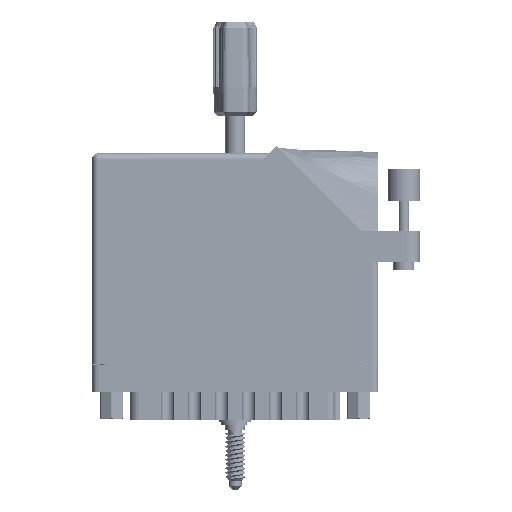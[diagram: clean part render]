
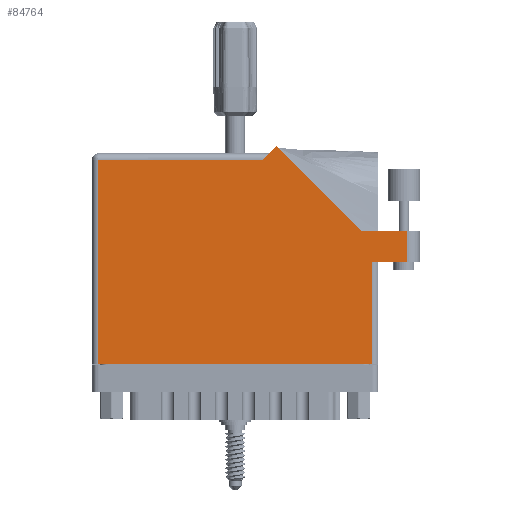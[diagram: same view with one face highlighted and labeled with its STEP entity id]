
A CAD part, front view. The second image highlights one B-rep face of the part: STEP entity #84764.
In plain terms, the highlighted face is planar.
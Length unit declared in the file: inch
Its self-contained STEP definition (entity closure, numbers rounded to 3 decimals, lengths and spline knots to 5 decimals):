
#1753 = CARTESIAN_POINT ( 'NONE',  ( 2.58942, 1.287, 0. ) ) ;
#4302 = EDGE_CURVE ( 'NONE', #12360, #84001, #58504, .T. ) ;
#6374 = LINE ( 'NONE', #61199, #70724 ) ;
#8116 = VERTEX_POINT ( 'NONE', #1753 ) ;
#9251 = VECTOR ( 'NONE', #90883, 39.37008 ) ;
#9544 = EDGE_CURVE ( 'NONE', #60245, #32958, #101732, .T. ) ;
#10695 = LINE ( 'NONE', #95578, #43067 ) ;
#12360 = VERTEX_POINT ( 'NONE', #118815 ) ;
#12663 = LINE ( 'NONE', #50572, #86017 ) ;
#13843 = CARTESIAN_POINT ( 'NONE',  ( 3.03, 0.98, 0. ) ) ;
#19299 = PLANE ( 'NONE',  #104740 ) ;
#20911 = CARTESIAN_POINT ( 'NONE',  ( 3.03, 1.287, 0. ) ) ;
#21012 = ORIENTED_EDGE ( 'NONE', *, *, #90095, .T. ) ;
#22523 = ORIENTED_EDGE ( 'NONE', *, *, #74579, .T. ) ;
#22728 = DIRECTION ( 'NONE',  ( 0., -1., 0. ) ) ;
#24081 = DIRECTION ( 'NONE',  ( 1., 0., 0. ) ) ;
#24288 = VECTOR ( 'NONE', #39299, 39.37008 ) ;
#24999 = VECTOR ( 'NONE', #111271, 39.37008 ) ;
#27294 = ORIENTED_EDGE ( 'NONE', *, *, #9544, .T. ) ;
#27380 = ORIENTED_EDGE ( 'NONE', *, *, #41243, .T. ) ;
#28600 = ORIENTED_EDGE ( 'NONE', *, *, #4302, .T. ) ;
#28712 = ORIENTED_EDGE ( 'NONE', *, *, #85772, .T. ) ;
#30125 = EDGE_CURVE ( 'NONE', #8116, #107748, #12663, .T. ) ;
#32958 = VERTEX_POINT ( 'NONE', #65084 ) ;
#33224 = VERTEX_POINT ( 'NONE', #13843 ) ;
#35771 = VECTOR ( 'NONE', #36540, 39.37008 ) ;
#36492 = LINE ( 'NONE', #65334, #107115 ) ;
#36540 = DIRECTION ( 'NONE',  ( -0.707, -0.707, 0. ) ) ;
#36702 = CARTESIAN_POINT ( 'NONE',  ( 0., 1.968, 0. ) ) ;
#37723 = CARTESIAN_POINT ( 'NONE',  ( 1.705, 2.03, 0. ) ) ;
#39299 = DIRECTION ( 'NONE',  ( 0., 1., 0. ) ) ;
#41243 = EDGE_CURVE ( 'NONE', #33224, #112738, #103423, .T. ) ;
#41567 = DIRECTION ( 'NONE',  ( -0.707, 0.707, 0. ) ) ;
#43067 = VECTOR ( 'NONE', #22728, 39.37008 ) ;
#43140 = DIRECTION ( 'NONE',  ( 1., 0., 0. ) ) ;
#45536 = VECTOR ( 'NONE', #24081, 39.37008 ) ;
#45822 = CARTESIAN_POINT ( 'NONE',  ( 0., 2.03, 0. ) ) ;
#47607 = DIRECTION ( 'NONE',  ( 0., 0., -1. ) ) ;
#50572 = CARTESIAN_POINT ( 'NONE',  ( 2.58942, 1.287, 0. ) ) ;
#51771 = CARTESIAN_POINT ( 'NONE',  ( 2.755, 0.98, 0. ) ) ;
#54120 = LINE ( 'NONE', #51771, #45536 ) ;
#58504 = LINE ( 'NONE', #94659, #24288 ) ;
#60245 = VERTEX_POINT ( 'NONE', #64465 ) ;
#61127 = EDGE_CURVE ( 'NONE', #107748, #60245, #119060, .T. ) ;
#61199 = CARTESIAN_POINT ( 'NONE',  ( 0., 0., 0. ) ) ;
#63850 = FACE_OUTER_BOUND ( 'NONE', #94912, .T. ) ;
#64465 = CARTESIAN_POINT ( 'NONE',  ( 1.643, 1.968, 0. ) ) ;
#65084 = CARTESIAN_POINT ( 'NONE',  ( 0.062, 1.968, 0. ) ) ;
#65334 = CARTESIAN_POINT ( 'NONE',  ( 3.155, 1.287, 0. ) ) ;
#67859 = CARTESIAN_POINT ( 'NONE',  ( 2.693, 0.98, 0. ) ) ;
#70724 = VECTOR ( 'NONE', #43140, 39.37008 ) ;
#74579 = EDGE_CURVE ( 'NONE', #84001, #33224, #54120, .T. ) ;
#82983 = CARTESIAN_POINT ( 'NONE',  ( 0.062, 0., 0. ) ) ;
#84001 = VERTEX_POINT ( 'NONE', #67859 ) ;
#84017 = DIRECTION ( 'NONE',  ( -1., 0., 0. ) ) ;
#84764 = ADVANCED_FACE ( 'NONE', ( #63850 ), #19299, .F. ) ;
#84846 = ORIENTED_EDGE ( 'NONE', *, *, #111519, .T. ) ;
#85772 = EDGE_CURVE ( 'NONE', #32958, #109943, #10695, .T. ) ;
#86017 = VECTOR ( 'NONE', #41567, 39.37008 ) ;
#90095 = EDGE_CURVE ( 'NONE', #109943, #12360, #6374, .T. ) ;
#90883 = DIRECTION ( 'NONE',  ( -1., 0., 0. ) ) ;
#92785 = CARTESIAN_POINT ( 'NONE',  ( 1.77571, 2.10071, 0. ) ) ;
#94659 = CARTESIAN_POINT ( 'NONE',  ( 2.693, 0.98, 0. ) ) ;
#94912 = EDGE_LOOP ( 'NONE', ( #22523, #27380, #84846, #117253, #110585, #27294, #28712, #21012, #28600 ) ) ;
#95578 = CARTESIAN_POINT ( 'NONE',  ( 0.062, 0., 0. ) ) ;
#101732 = LINE ( 'NONE', #36702, #9251 ) ;
#103327 = CARTESIAN_POINT ( 'NONE',  ( 3.03, 1.287, 0. ) ) ;
#103423 = LINE ( 'NONE', #20911, #24999 ) ;
#104740 = AXIS2_PLACEMENT_3D ( 'NONE', #45822, #47607, #112050 ) ;
#107115 = VECTOR ( 'NONE', #84017, 39.37008 ) ;
#107748 = VERTEX_POINT ( 'NONE', #92785 ) ;
#109943 = VERTEX_POINT ( 'NONE', #82983 ) ;
#110585 = ORIENTED_EDGE ( 'NONE', *, *, #61127, .T. ) ;
#111271 = DIRECTION ( 'NONE',  ( 0., 1., 0. ) ) ;
#111519 = EDGE_CURVE ( 'NONE', #112738, #8116, #36492, .T. ) ;
#112050 = DIRECTION ( 'NONE',  ( -1., 0., 0. ) ) ;
#112738 = VERTEX_POINT ( 'NONE', #103327 ) ;
#117253 = ORIENTED_EDGE ( 'NONE', *, *, #30125, .T. ) ;
#118815 = CARTESIAN_POINT ( 'NONE',  ( 2.693, 0., 0. ) ) ;
#119060 = LINE ( 'NONE', #37723, #35771 ) ;
